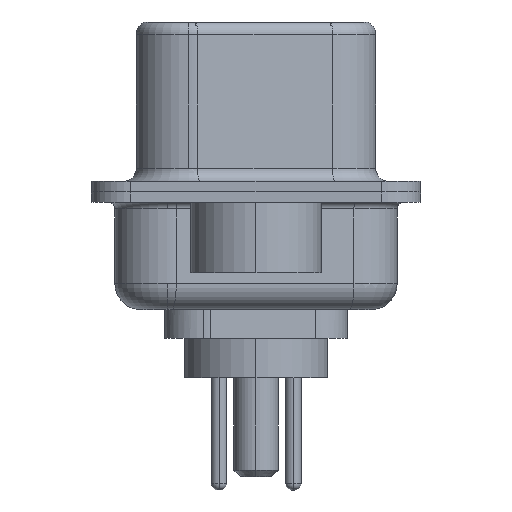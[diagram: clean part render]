
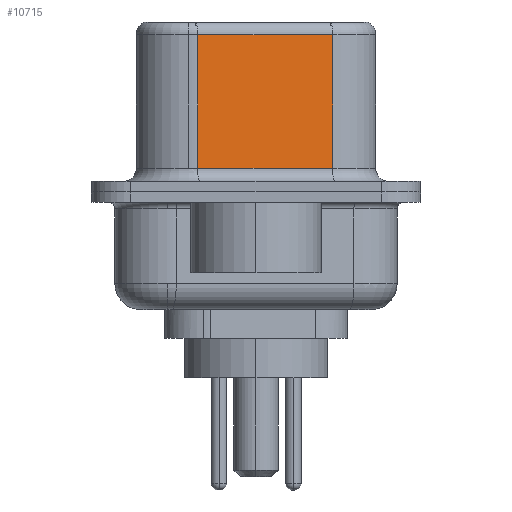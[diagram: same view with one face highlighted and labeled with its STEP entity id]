
A CAD part, left-side view. The second image highlights one B-rep face of the part: STEP entity #10715.
In plain terms, the highlighted planar face has unit normal (-0.985, -0.174, 0).
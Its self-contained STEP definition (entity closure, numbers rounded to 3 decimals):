
#253 = DIRECTION ( 'NONE',  ( -0.174, 0.985, 0. ) ) ;
#709 = ORIENTED_EDGE ( 'NONE', *, *, #1742, .T. ) ;
#771 = VECTOR ( 'NONE', #1617, 1000. ) ;
#1435 = EDGE_CURVE ( 'NONE', #1657, #13584, #13950, .T. ) ;
#1617 = DIRECTION ( 'NONE',  ( 0.174, -0.985, 0. ) ) ;
#1657 = VERTEX_POINT ( 'NONE', #3341 ) ;
#1742 = EDGE_CURVE ( 'NONE', #11525, #1657, #17211, .T. ) ;
#1977 = CARTESIAN_POINT ( 'NONE',  ( 4.58, -2.927, 6.02 ) ) ;
#3341 = CARTESIAN_POINT ( 'NONE',  ( 3.67, 2.233, 0.9 ) ) ;
#3785 = CARTESIAN_POINT ( 'NONE',  ( 4.58, -2.927, 6.52 ) ) ;
#3827 = EDGE_CURVE ( 'NONE', #8631, #13584, #15451, .T. ) ;
#4353 = EDGE_CURVE ( 'NONE', #8631, #11525, #23225, .T. ) ;
#6816 = DIRECTION ( 'NONE',  ( 0.985, 0.174, 0. ) ) ;
#8305 = DIRECTION ( 'NONE',  ( 0., 0., -1. ) ) ;
#8631 = VERTEX_POINT ( 'NONE', #17605 ) ;
#10642 = CARTESIAN_POINT ( 'NONE',  ( 3.67, 2.233, 6.52 ) ) ;
#10715 = ADVANCED_FACE ( 'NONE', ( #12649 ), #17403, .F. ) ;
#10719 = CARTESIAN_POINT ( 'NONE',  ( 3.67, 2.233, 6.02 ) ) ;
#11525 = VERTEX_POINT ( 'NONE', #10719 ) ;
#11935 = ORIENTED_EDGE ( 'NONE', *, *, #4353, .T. ) ;
#12058 = CARTESIAN_POINT ( 'NONE',  ( 4.58, -2.927, 0.9 ) ) ;
#12519 = VECTOR ( 'NONE', #8305, 1000. ) ;
#12649 = FACE_OUTER_BOUND ( 'NONE', #23104, .T. ) ;
#13338 = CARTESIAN_POINT ( 'NONE',  ( 4.58, -2.927, 6.52 ) ) ;
#13584 = VERTEX_POINT ( 'NONE', #12058 ) ;
#13950 = LINE ( 'NONE', #20396, #771 ) ;
#15451 = LINE ( 'NONE', #3785, #19531 ) ;
#17211 = LINE ( 'NONE', #10642, #12519 ) ;
#17403 = PLANE ( 'NONE',  #20099 ) ;
#17605 = CARTESIAN_POINT ( 'NONE',  ( 4.58, -2.927, 6.02 ) ) ;
#18385 = VECTOR ( 'NONE', #253, 1000. ) ;
#18888 = ORIENTED_EDGE ( 'NONE', *, *, #1435, .T. ) ;
#19192 = DIRECTION ( 'NONE',  ( -0.174, 0.985, 0. ) ) ;
#19531 = VECTOR ( 'NONE', #20483, 1000. ) ;
#20099 = AXIS2_PLACEMENT_3D ( 'NONE', #13338, #6816, #19192 ) ;
#20396 = CARTESIAN_POINT ( 'NONE',  ( 4.58, -2.927, 0.9 ) ) ;
#20483 = DIRECTION ( 'NONE',  ( 0., 0., -1. ) ) ;
#22764 = ORIENTED_EDGE ( 'NONE', *, *, #3827, .F. ) ;
#23104 = EDGE_LOOP ( 'NONE', ( #22764, #11935, #709, #18888 ) ) ;
#23225 = LINE ( 'NONE', #1977, #18385 ) ;
